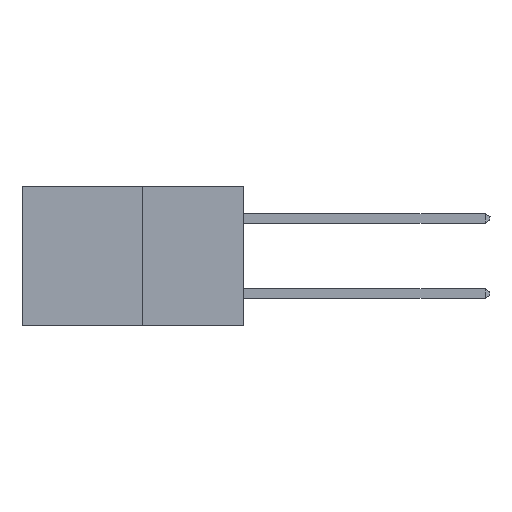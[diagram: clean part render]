
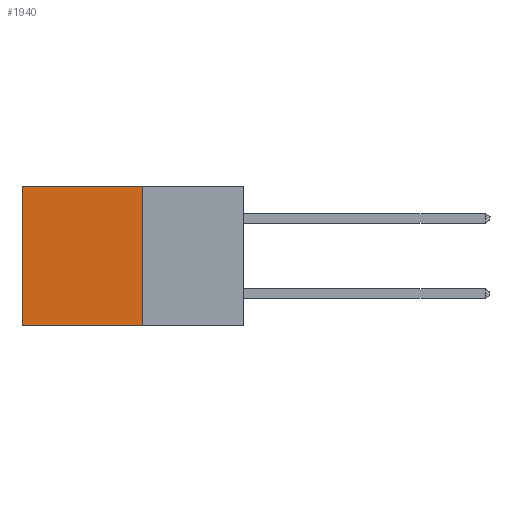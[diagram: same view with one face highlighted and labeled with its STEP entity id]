
A CAD part, left-side view. The second image highlights one B-rep face of the part: STEP entity #1940.
In plain terms, the highlighted planar face has unit normal (-1, 0, 0).
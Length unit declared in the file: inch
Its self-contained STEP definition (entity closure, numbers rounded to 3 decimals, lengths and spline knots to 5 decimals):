
#106 = VERTEX_POINT ( 'NONE', #7404 ) ;
#144 = EDGE_CURVE ( 'NONE', #106, #4031, #7712, .T. ) ;
#663 = EDGE_CURVE ( 'NONE', #106, #3454, #7705, .T. ) ;
#1245 = FACE_OUTER_BOUND ( 'NONE', #3566, .T. ) ;
#1460 = ORIENTED_EDGE ( 'NONE', *, *, #4332, .T. ) ;
#1513 = DIRECTION ( 'NONE',  ( 0., 1., 0. ) ) ;
#1552 = LINE ( 'NONE', #4437, #6246 ) ;
#1622 = EDGE_CURVE ( 'NONE', #4031, #2630, #1552, .T. ) ;
#1798 = PLANE ( 'NONE',  #6923 ) ;
#1813 = ORIENTED_EDGE ( 'NONE', *, *, #1622, .F. ) ;
#1940 = ADVANCED_FACE ( 'NONE', ( #1245 ), #1798, .F. ) ;
#2311 = VECTOR ( 'NONE', #5310, 39.37008 ) ;
#2498 = LINE ( 'NONE', #5038, #2311 ) ;
#2630 = VERTEX_POINT ( 'NONE', #6429 ) ;
#3375 = DIRECTION ( 'NONE',  ( 0., 0., -1. ) ) ;
#3454 = VERTEX_POINT ( 'NONE', #6798 ) ;
#3483 = CARTESIAN_POINT ( 'NONE',  ( 0.277, 0.27, -0.37 ) ) ;
#3507 = DIRECTION ( 'NONE',  ( 0., 0., -1. ) ) ;
#3566 = EDGE_LOOP ( 'NONE', ( #1460, #1813, #7033, #6193 ) ) ;
#3889 = CARTESIAN_POINT ( 'NONE',  ( 0.277, 0.27, 0. ) ) ;
#4031 = VERTEX_POINT ( 'NONE', #4530 ) ;
#4332 = EDGE_CURVE ( 'NONE', #3454, #2630, #2498, .T. ) ;
#4437 = CARTESIAN_POINT ( 'NONE',  ( 0.277, 0.27, -0.37 ) ) ;
#4530 = CARTESIAN_POINT ( 'NONE',  ( 0.277, 0.27, -0.37 ) ) ;
#4647 = CARTESIAN_POINT ( 'NONE',  ( 0.277, 0.27, -0.37 ) ) ;
#4794 = VECTOR ( 'NONE', #3507, 39.37008 ) ;
#5038 = CARTESIAN_POINT ( 'NONE',  ( 0.277, 0.59, -0.37 ) ) ;
#5310 = DIRECTION ( 'NONE',  ( 0., 0., -1. ) ) ;
#6169 = VECTOR ( 'NONE', #7462, 39.37008 ) ;
#6193 = ORIENTED_EDGE ( 'NONE', *, *, #663, .T. ) ;
#6246 = VECTOR ( 'NONE', #1513, 39.37008 ) ;
#6429 = CARTESIAN_POINT ( 'NONE',  ( 0.277, 0.59, -0.37 ) ) ;
#6798 = CARTESIAN_POINT ( 'NONE',  ( 0.277, 0.59, 0. ) ) ;
#6923 = AXIS2_PLACEMENT_3D ( 'NONE', #4647, #7735, #3375 ) ;
#7033 = ORIENTED_EDGE ( 'NONE', *, *, #144, .F. ) ;
#7404 = CARTESIAN_POINT ( 'NONE',  ( 0.277, 0.27, 0. ) ) ;
#7462 = DIRECTION ( 'NONE',  ( 0., 1., 0. ) ) ;
#7705 = LINE ( 'NONE', #3889, #6169 ) ;
#7712 = LINE ( 'NONE', #3483, #4794 ) ;
#7735 = DIRECTION ( 'NONE',  ( 1., 0., 0. ) ) ;
